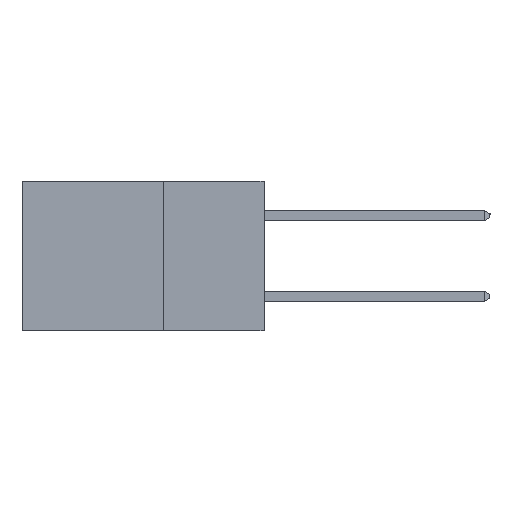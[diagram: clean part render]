
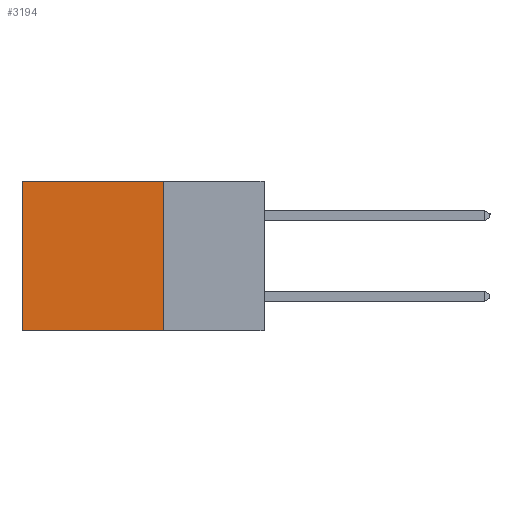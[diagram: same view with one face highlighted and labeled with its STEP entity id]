
A CAD part, left-side view. The second image highlights one B-rep face of the part: STEP entity #3194.
In plain terms, the highlighted planar face has unit normal (-1, 0, 0).
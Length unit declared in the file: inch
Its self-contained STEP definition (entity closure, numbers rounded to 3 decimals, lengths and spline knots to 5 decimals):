
#279 = FACE_OUTER_BOUND ( 'NONE', #6080, .T. ) ;
#428 = DIRECTION ( 'NONE',  ( 1., 0., 0. ) ) ;
#774 = CARTESIAN_POINT ( 'NONE',  ( 0.2615, 0.25, -0.37 ) ) ;
#992 = LINE ( 'NONE', #8074, #10130 ) ;
#1571 = CARTESIAN_POINT ( 'NONE',  ( 0.2615, 0.25, -0.37 ) ) ;
#1732 = CARTESIAN_POINT ( 'NONE',  ( 0.2615, 0.25, -0.37 ) ) ;
#1775 = AXIS2_PLACEMENT_3D ( 'NONE', #2660, #428, #13999 ) ;
#1816 = DIRECTION ( 'NONE',  ( 0., 0., -1. ) ) ;
#1926 = CARTESIAN_POINT ( 'NONE',  ( 0.2615, 0.6, 0. ) ) ;
#2660 = CARTESIAN_POINT ( 'NONE',  ( 0.2615, 0.25, -0.37 ) ) ;
#2902 = DIRECTION ( 'NONE',  ( 0., 1., 0. ) ) ;
#3194 = ADVANCED_FACE ( 'NONE', ( #279 ), #12895, .F. ) ;
#3688 = VERTEX_POINT ( 'NONE', #1732 ) ;
#4951 = EDGE_CURVE ( 'NONE', #12102, #7953, #11692, .T. ) ;
#5533 = ORIENTED_EDGE ( 'NONE', *, *, #4951, .T. ) ;
#6080 = EDGE_LOOP ( 'NONE', ( #5533, #8742, #9816, #7423 ) ) ;
#6154 = VERTEX_POINT ( 'NONE', #6970 ) ;
#6196 = LINE ( 'NONE', #1571, #10410 ) ;
#6970 = CARTESIAN_POINT ( 'NONE',  ( 0.2615, 0.25, 0. ) ) ;
#7072 = EDGE_CURVE ( 'NONE', #3688, #7953, #6196, .T. ) ;
#7423 = ORIENTED_EDGE ( 'NONE', *, *, #9420, .T. ) ;
#7854 = DIRECTION ( 'NONE',  ( 0., 1., 0. ) ) ;
#7953 = VERTEX_POINT ( 'NONE', #13916 ) ;
#8049 = VECTOR ( 'NONE', #1816, 39.37008 ) ;
#8074 = CARTESIAN_POINT ( 'NONE',  ( 0.2615, 0.25, 0. ) ) ;
#8235 = CARTESIAN_POINT ( 'NONE',  ( 0.2615, 0.6, -0.37 ) ) ;
#8742 = ORIENTED_EDGE ( 'NONE', *, *, #7072, .F. ) ;
#9420 = EDGE_CURVE ( 'NONE', #6154, #12102, #992, .T. ) ;
#9816 = ORIENTED_EDGE ( 'NONE', *, *, #13010, .F. ) ;
#10130 = VECTOR ( 'NONE', #7854, 39.37008 ) ;
#10369 = VECTOR ( 'NONE', #11981, 39.37008 ) ;
#10410 = VECTOR ( 'NONE', #2902, 39.37008 ) ;
#11692 = LINE ( 'NONE', #8235, #10369 ) ;
#11981 = DIRECTION ( 'NONE',  ( 0., 0., -1. ) ) ;
#12102 = VERTEX_POINT ( 'NONE', #1926 ) ;
#12358 = LINE ( 'NONE', #774, #8049 ) ;
#12895 = PLANE ( 'NONE',  #1775 ) ;
#13010 = EDGE_CURVE ( 'NONE', #6154, #3688, #12358, .T. ) ;
#13916 = CARTESIAN_POINT ( 'NONE',  ( 0.2615, 0.6, -0.37 ) ) ;
#13999 = DIRECTION ( 'NONE',  ( 0., 0., -1. ) ) ;
